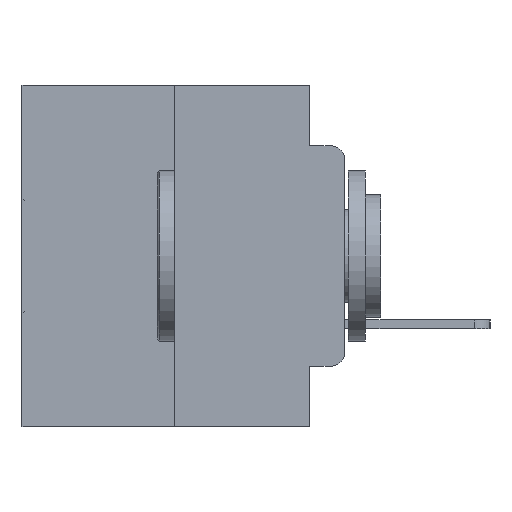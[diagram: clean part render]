
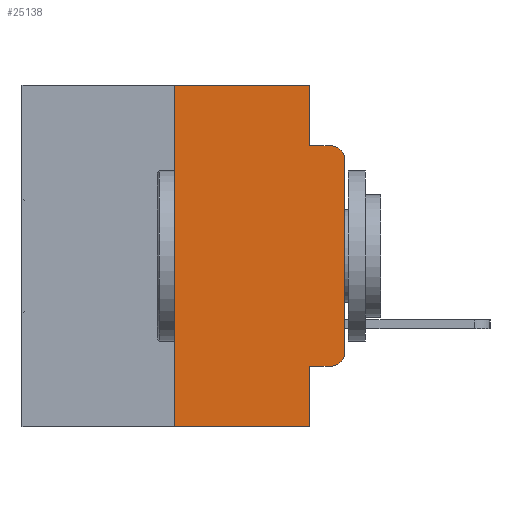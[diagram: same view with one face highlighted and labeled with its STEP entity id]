
A CAD part, left-side view. The second image highlights one B-rep face of the part: STEP entity #25138.
In plain terms, the highlighted planar face has unit normal (-1, 0, 0).
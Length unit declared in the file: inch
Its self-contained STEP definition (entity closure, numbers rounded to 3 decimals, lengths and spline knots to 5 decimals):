
#408 = CIRCLE ( 'NONE', #21664, 0.02 ) ;
#943 = EDGE_CURVE ( 'NONE', #25321, #10106, #12172, .T. ) ;
#1042 = CARTESIAN_POINT ( 'NONE',  ( 0., 0.051, 0. ) ) ;
#2630 = EDGE_CURVE ( 'NONE', #10106, #11110, #5414, .T. ) ;
#3265 = DIRECTION ( 'NONE',  ( -1., 0., 0. ) ) ;
#3499 = CARTESIAN_POINT ( 'NONE',  ( 0., 0.02, -0.1085 ) ) ;
#4271 = EDGE_CURVE ( 'NONE', #6788, #11110, #24084, .T. ) ;
#4918 = DIRECTION ( 'NONE',  ( 0., -1., 0. ) ) ;
#5058 = CARTESIAN_POINT ( 'NONE',  ( 0., 0.051, -0.0885 ) ) ;
#5414 = LINE ( 'NONE', #5058, #29211 ) ;
#5744 = LINE ( 'NONE', #11214, #18046 ) ;
#5873 = EDGE_CURVE ( 'NONE', #26585, #6788, #22739, .T. ) ;
#6095 = CARTESIAN_POINT ( 'NONE',  ( 0., 0.051, -0.0885 ) ) ;
#6371 = DIRECTION ( 'NONE',  ( -1., 0., 0. ) ) ;
#6476 = EDGE_CURVE ( 'NONE', #7541, #26585, #408, .T. ) ;
#6530 = DIRECTION ( 'NONE',  ( 0., 0., -1. ) ) ;
#6671 = DIRECTION ( 'NONE',  ( 0., 0., -1. ) ) ;
#6788 = VERTEX_POINT ( 'NONE', #6855 ) ;
#6855 = CARTESIAN_POINT ( 'NONE',  ( 0., 0., -0.1085 ) ) ;
#7541 = VERTEX_POINT ( 'NONE', #26353 ) ;
#7782 = DIRECTION ( 'NONE',  ( 0., 0., -1. ) ) ;
#7871 = ORIENTED_EDGE ( 'NONE', *, *, #17304, .T. ) ;
#8272 = DIRECTION ( 'NONE',  ( 0., 0., 1. ) ) ;
#8608 = ORIENTED_EDGE ( 'NONE', *, *, #6476, .T. ) ;
#8979 = ORIENTED_EDGE ( 'NONE', *, *, #5873, .T. ) ;
#9586 = DIRECTION ( 'NONE',  ( 0., -1., 0. ) ) ;
#9963 = VECTOR ( 'NONE', #8272, 39.37008 ) ;
#10106 = VERTEX_POINT ( 'NONE', #6095 ) ;
#10400 = LINE ( 'NONE', #27676, #21761 ) ;
#10452 = ORIENTED_EDGE ( 'NONE', *, *, #2630, .F. ) ;
#11110 = VERTEX_POINT ( 'NONE', #27443 ) ;
#11214 = CARTESIAN_POINT ( 'NONE',  ( 0., 0.051, -0.4115 ) ) ;
#11238 = CARTESIAN_POINT ( 'NONE',  ( 0., 0.051, -0.4115 ) ) ;
#11920 = CARTESIAN_POINT ( 'NONE',  ( 0., 0.25, -0.5 ) ) ;
#12172 = LINE ( 'NONE', #21648, #12864 ) ;
#12582 = ORIENTED_EDGE ( 'NONE', *, *, #18828, .F. ) ;
#12864 = VECTOR ( 'NONE', #15835, 39.37008 ) ;
#13531 = VERTEX_POINT ( 'NONE', #11920 ) ;
#14060 = CARTESIAN_POINT ( 'NONE',  ( 0., 0.473, 0. ) ) ;
#14590 = VERTEX_POINT ( 'NONE', #22967 ) ;
#14617 = PLANE ( 'NONE',  #29006 ) ;
#15010 = LINE ( 'NONE', #14060, #27175 ) ;
#15048 = EDGE_CURVE ( 'NONE', #13531, #24654, #15748, .T. ) ;
#15687 = CARTESIAN_POINT ( 'NONE',  ( 0., 0.473, -0.5 ) ) ;
#15748 = LINE ( 'NONE', #15687, #20382 ) ;
#15835 = DIRECTION ( 'NONE',  ( 0., 0., -1. ) ) ;
#16469 = ORIENTED_EDGE ( 'NONE', *, *, #943, .F. ) ;
#17235 = CARTESIAN_POINT ( 'NONE',  ( 0., 0.02, -0.3915 ) ) ;
#17304 = EDGE_CURVE ( 'NONE', #18579, #7541, #5744, .T. ) ;
#17370 = CARTESIAN_POINT ( 'NONE',  ( 0., 0., 0. ) ) ;
#17904 = ORIENTED_EDGE ( 'NONE', *, *, #20359, .F. ) ;
#18046 = VECTOR ( 'NONE', #27162, 39.37008 ) ;
#18579 = VERTEX_POINT ( 'NONE', #11238 ) ;
#18637 = EDGE_LOOP ( 'NONE', ( #8979, #21102, #10452, #16469, #28686, #17904, #23988, #12582, #7871, #8608 ) ) ;
#18828 = EDGE_CURVE ( 'NONE', #18579, #24654, #29790, .T. ) ;
#19516 = DIRECTION ( 'NONE',  ( 0., 0., -1. ) ) ;
#19809 = CARTESIAN_POINT ( 'NONE',  ( 0., 0.051, -0.5 ) ) ;
#20359 = EDGE_CURVE ( 'NONE', #13531, #14590, #10400, .T. ) ;
#20382 = VECTOR ( 'NONE', #29409, 39.37008 ) ;
#20405 = EDGE_CURVE ( 'NONE', #14590, #25321, #15010, .T. ) ;
#21102 = ORIENTED_EDGE ( 'NONE', *, *, #4271, .T. ) ;
#21479 = DIRECTION ( 'NONE',  ( 1., 0., 0. ) ) ;
#21648 = CARTESIAN_POINT ( 'NONE',  ( 0., 0.051, 0. ) ) ;
#21664 = AXIS2_PLACEMENT_3D ( 'NONE', #17235, #3265, #19516 ) ;
#21761 = VECTOR ( 'NONE', #27580, 39.37008 ) ;
#21847 = CARTESIAN_POINT ( 'NONE',  ( 0., 0., -0.3915 ) ) ;
#22739 = LINE ( 'NONE', #17370, #9963 ) ;
#22918 = VECTOR ( 'NONE', #6530, 39.37008 ) ;
#22967 = CARTESIAN_POINT ( 'NONE',  ( 0., 0.25, 0. ) ) ;
#23988 = ORIENTED_EDGE ( 'NONE', *, *, #15048, .T. ) ;
#24084 = CIRCLE ( 'NONE', #25888, 0.02 ) ;
#24654 = VERTEX_POINT ( 'NONE', #19809 ) ;
#24926 = CARTESIAN_POINT ( 'NONE',  ( 0., 0.051, 0. ) ) ;
#25138 = ADVANCED_FACE ( 'NONE', ( #28801 ), #14617, .F. ) ;
#25321 = VERTEX_POINT ( 'NONE', #1042 ) ;
#25888 = AXIS2_PLACEMENT_3D ( 'NONE', #3499, #6371, #6671 ) ;
#26004 = CARTESIAN_POINT ( 'NONE',  ( 0., 0.473, 0. ) ) ;
#26353 = CARTESIAN_POINT ( 'NONE',  ( 0., 0.02, -0.4115 ) ) ;
#26585 = VERTEX_POINT ( 'NONE', #21847 ) ;
#27162 = DIRECTION ( 'NONE',  ( 0., -1., 0. ) ) ;
#27175 = VECTOR ( 'NONE', #9586, 39.37008 ) ;
#27443 = CARTESIAN_POINT ( 'NONE',  ( 0., 0.02, -0.0885 ) ) ;
#27580 = DIRECTION ( 'NONE',  ( 0., 0., 1. ) ) ;
#27676 = CARTESIAN_POINT ( 'NONE',  ( 0., 0.25, 0. ) ) ;
#28686 = ORIENTED_EDGE ( 'NONE', *, *, #20405, .F. ) ;
#28801 = FACE_OUTER_BOUND ( 'NONE', #18637, .T. ) ;
#29006 = AXIS2_PLACEMENT_3D ( 'NONE', #26004, #21479, #7782 ) ;
#29211 = VECTOR ( 'NONE', #4918, 39.37008 ) ;
#29409 = DIRECTION ( 'NONE',  ( 0., -1., 0. ) ) ;
#29790 = LINE ( 'NONE', #24926, #22918 ) ;
